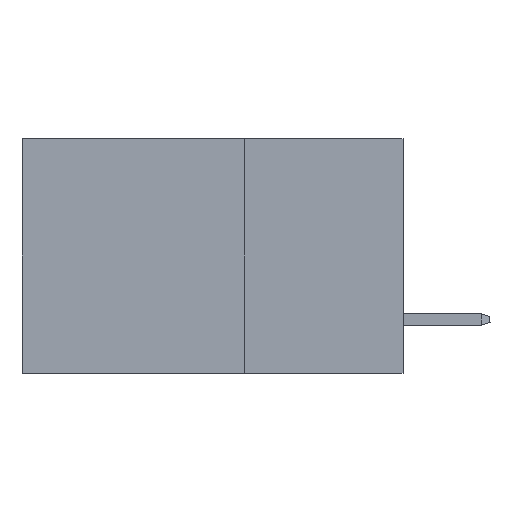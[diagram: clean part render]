
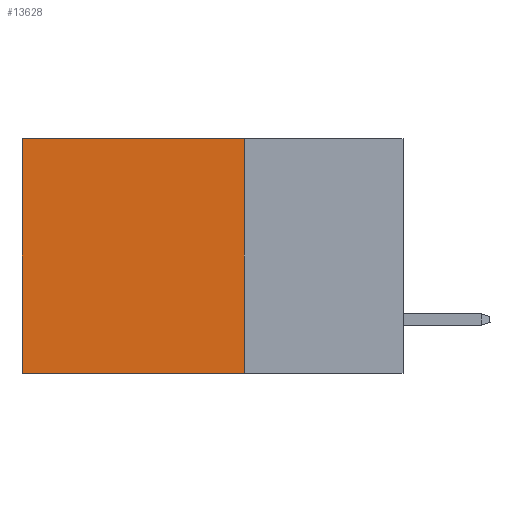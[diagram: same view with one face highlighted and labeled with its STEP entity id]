
A CAD part, left-side view. The second image highlights one B-rep face of the part: STEP entity #13628.
In plain terms, the highlighted planar face has unit normal (-1, 0, 0).
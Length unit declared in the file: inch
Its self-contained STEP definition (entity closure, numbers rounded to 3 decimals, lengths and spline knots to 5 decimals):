
#291 = CARTESIAN_POINT ( 'NONE',  ( 0.2875, 0.6, 0. ) ) ;
#558 = DIRECTION ( 'NONE',  ( 0., 0., -1. ) ) ;
#610 = CARTESIAN_POINT ( 'NONE',  ( 0.2875, 0.25, 0. ) ) ;
#1300 = CARTESIAN_POINT ( 'NONE',  ( 0.2875, 0.25, -0.37 ) ) ;
#1816 = EDGE_CURVE ( 'NONE', #18477, #13452, #10779, .T. ) ;
#2141 = VECTOR ( 'NONE', #21879, 39.37008 ) ;
#2252 = CARTESIAN_POINT ( 'NONE',  ( 0.2875, 0.6, 0. ) ) ;
#4290 = LINE ( 'NONE', #2252, #13843 ) ;
#4702 = EDGE_CURVE ( 'NONE', #13452, #7967, #10156, .T. ) ;
#5786 = CARTESIAN_POINT ( 'NONE',  ( 0.2875, 0.25, -0.37 ) ) ;
#7920 = DIRECTION ( 'NONE',  ( 0., 0., -1. ) ) ;
#7967 = VERTEX_POINT ( 'NONE', #17625 ) ;
#8158 = DIRECTION ( 'NONE',  ( 1., 0., 0. ) ) ;
#8767 = AXIS2_PLACEMENT_3D ( 'NONE', #610, #8158, #7920 ) ;
#9435 = ORIENTED_EDGE ( 'NONE', *, *, #20480, .T. ) ;
#9703 = FACE_OUTER_BOUND ( 'NONE', #16161, .T. ) ;
#10156 = LINE ( 'NONE', #1300, #18826 ) ;
#10395 = ORIENTED_EDGE ( 'NONE', *, *, #16828, .T. ) ;
#10779 = LINE ( 'NONE', #12447, #15928 ) ;
#12447 = CARTESIAN_POINT ( 'NONE',  ( 0.2875, 0.25, 0. ) ) ;
#13452 = VERTEX_POINT ( 'NONE', #5786 ) ;
#13628 = ADVANCED_FACE ( 'NONE', ( #9703 ), #16993, .F. ) ;
#13843 = VECTOR ( 'NONE', #558, 39.37008 ) ;
#15928 = VECTOR ( 'NONE', #18426, 39.37008 ) ;
#16161 = EDGE_LOOP ( 'NONE', ( #10395, #19092, #16486, #9435 ) ) ;
#16486 = ORIENTED_EDGE ( 'NONE', *, *, #1816, .F. ) ;
#16828 = EDGE_CURVE ( 'NONE', #21097, #7967, #4290, .T. ) ;
#16993 = PLANE ( 'NONE',  #8767 ) ;
#17563 = DIRECTION ( 'NONE',  ( 0., 1., 0. ) ) ;
#17625 = CARTESIAN_POINT ( 'NONE',  ( 0.2875, 0.6, -0.37 ) ) ;
#18153 = LINE ( 'NONE', #20315, #2141 ) ;
#18426 = DIRECTION ( 'NONE',  ( 0., 0., -1. ) ) ;
#18477 = VERTEX_POINT ( 'NONE', #20103 ) ;
#18826 = VECTOR ( 'NONE', #17563, 39.37008 ) ;
#19092 = ORIENTED_EDGE ( 'NONE', *, *, #4702, .F. ) ;
#20103 = CARTESIAN_POINT ( 'NONE',  ( 0.2875, 0.25, 0. ) ) ;
#20315 = CARTESIAN_POINT ( 'NONE',  ( 0.2875, 0.25, 0. ) ) ;
#20480 = EDGE_CURVE ( 'NONE', #18477, #21097, #18153, .T. ) ;
#21097 = VERTEX_POINT ( 'NONE', #291 ) ;
#21879 = DIRECTION ( 'NONE',  ( 0., 1., 0. ) ) ;
